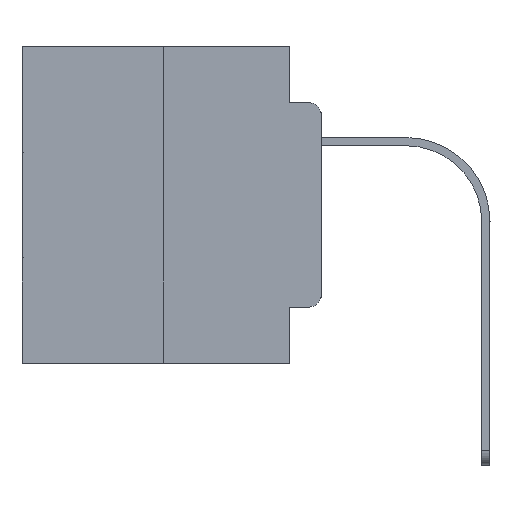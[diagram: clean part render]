
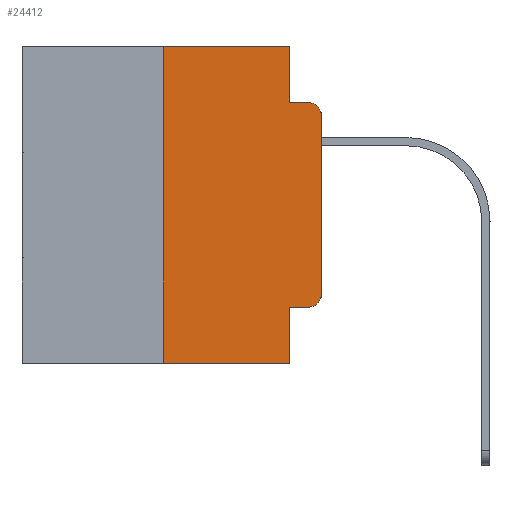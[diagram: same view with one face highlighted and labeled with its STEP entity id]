
A CAD part, left-side view. The second image highlights one B-rep face of the part: STEP entity #24412.
In plain terms, the highlighted planar face has unit normal (-1, 0, 0).
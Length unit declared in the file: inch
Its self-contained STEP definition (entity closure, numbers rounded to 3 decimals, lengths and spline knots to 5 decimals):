
#120 = CARTESIAN_POINT ( 'NONE',  ( 0., 0.051, -0.5 ) ) ;
#206 = ORIENTED_EDGE ( 'NONE', *, *, #8488, .T. ) ;
#531 = DIRECTION ( 'NONE',  ( 0., 0., -1. ) ) ;
#1294 = EDGE_CURVE ( 'NONE', #10812, #5511, #18435, .T. ) ;
#1433 = CARTESIAN_POINT ( 'NONE',  ( 0., 0.051, -0.4115 ) ) ;
#1598 = VERTEX_POINT ( 'NONE', #1433 ) ;
#1786 = CARTESIAN_POINT ( 'NONE',  ( 0., 0.02, -0.3915 ) ) ;
#2183 = DIRECTION ( 'NONE',  ( 1., 0., 0. ) ) ;
#2204 = DIRECTION ( 'NONE',  ( 0., 0., 1. ) ) ;
#2426 = VECTOR ( 'NONE', #15109, 39.37008 ) ;
#2468 = LINE ( 'NONE', #6788, #6600 ) ;
#2568 = DIRECTION ( 'NONE',  ( 0., -1., 0. ) ) ;
#2831 = DIRECTION ( 'NONE',  ( 0., -1., 0. ) ) ;
#2856 = LINE ( 'NONE', #23147, #14906 ) ;
#3822 = ORIENTED_EDGE ( 'NONE', *, *, #11584, .F. ) ;
#3892 = VERTEX_POINT ( 'NONE', #4068 ) ;
#4068 = CARTESIAN_POINT ( 'NONE',  ( 0., 0., -0.3915 ) ) ;
#4107 = DIRECTION ( 'NONE',  ( 0., 0., -1. ) ) ;
#4409 = VECTOR ( 'NONE', #6607, 39.37008 ) ;
#4613 = PLANE ( 'NONE',  #5698 ) ;
#5511 = VERTEX_POINT ( 'NONE', #15669 ) ;
#5698 = AXIS2_PLACEMENT_3D ( 'NONE', #10422, #2183, #10957 ) ;
#6008 = CARTESIAN_POINT ( 'NONE',  ( 0., 0.02, -0.1085 ) ) ;
#6032 = DIRECTION ( 'NONE',  ( 0., -1., 0. ) ) ;
#6600 = VECTOR ( 'NONE', #2204, 39.37008 ) ;
#6607 = DIRECTION ( 'NONE',  ( 0., 0., 1. ) ) ;
#6787 = EDGE_CURVE ( 'NONE', #10976, #25309, #18533, .T. ) ;
#6788 = CARTESIAN_POINT ( 'NONE',  ( 0., 0., 0. ) ) ;
#7060 = AXIS2_PLACEMENT_3D ( 'NONE', #6008, #7903, #4107 ) ;
#7903 = DIRECTION ( 'NONE',  ( -1., 0., 0. ) ) ;
#8488 = EDGE_CURVE ( 'NONE', #9969, #12125, #22486, .T. ) ;
#8764 = CARTESIAN_POINT ( 'NONE',  ( 0., 0.051, 0. ) ) ;
#8902 = EDGE_LOOP ( 'NONE', ( #17900, #206, #23940, #16121, #20036, #3822, #11712, #24834, #10517, #17631 ) ) ;
#9312 = LINE ( 'NONE', #17511, #2426 ) ;
#9969 = VERTEX_POINT ( 'NONE', #13968 ) ;
#10422 = CARTESIAN_POINT ( 'NONE',  ( 0., 0.473, 0. ) ) ;
#10517 = ORIENTED_EDGE ( 'NONE', *, *, #19918, .T. ) ;
#10812 = VERTEX_POINT ( 'NONE', #23879 ) ;
#10957 = DIRECTION ( 'NONE',  ( 0., 0., -1. ) ) ;
#10976 = VERTEX_POINT ( 'NONE', #13969 ) ;
#11100 = CARTESIAN_POINT ( 'NONE',  ( 0., 0.02, -0.4115 ) ) ;
#11236 = CIRCLE ( 'NONE', #21063, 0.02 ) ;
#11324 = VERTEX_POINT ( 'NONE', #19416 ) ;
#11584 = EDGE_CURVE ( 'NONE', #10976, #11324, #18857, .T. ) ;
#11661 = VECTOR ( 'NONE', #6032, 39.37008 ) ;
#11712 = ORIENTED_EDGE ( 'NONE', *, *, #6787, .T. ) ;
#12125 = VERTEX_POINT ( 'NONE', #23629 ) ;
#13400 = VECTOR ( 'NONE', #531, 39.37008 ) ;
#13942 = DIRECTION ( 'NONE',  ( -1., 0., 0. ) ) ;
#13968 = CARTESIAN_POINT ( 'NONE',  ( 0., 0., -0.1085 ) ) ;
#13969 = CARTESIAN_POINT ( 'NONE',  ( 0., 0.25, -0.5 ) ) ;
#14057 = VERTEX_POINT ( 'NONE', #11100 ) ;
#14059 = LINE ( 'NONE', #8764, #13400 ) ;
#14600 = EDGE_CURVE ( 'NONE', #3892, #9969, #2468, .T. ) ;
#14906 = VECTOR ( 'NONE', #2568, 39.37008 ) ;
#15109 = DIRECTION ( 'NONE',  ( 0., -1., 0. ) ) ;
#15669 = CARTESIAN_POINT ( 'NONE',  ( 0., 0.051, -0.0885 ) ) ;
#16121 = ORIENTED_EDGE ( 'NONE', *, *, #1294, .F. ) ;
#16690 = DIRECTION ( 'NONE',  ( 0., 0., -1. ) ) ;
#16880 = EDGE_CURVE ( 'NONE', #11324, #10812, #9312, .T. ) ;
#17511 = CARTESIAN_POINT ( 'NONE',  ( 0., 0.473, 0. ) ) ;
#17631 = ORIENTED_EDGE ( 'NONE', *, *, #22977, .T. ) ;
#17900 = ORIENTED_EDGE ( 'NONE', *, *, #14600, .T. ) ;
#18257 = EDGE_CURVE ( 'NONE', #5511, #12125, #2856, .T. ) ;
#18435 = LINE ( 'NONE', #20680, #21649 ) ;
#18533 = LINE ( 'NONE', #26464, #11661 ) ;
#18857 = LINE ( 'NONE', #20723, #4409 ) ;
#18967 = LINE ( 'NONE', #19107, #21801 ) ;
#19107 = CARTESIAN_POINT ( 'NONE',  ( 0., 0.051, -0.4115 ) ) ;
#19416 = CARTESIAN_POINT ( 'NONE',  ( 0., 0.25, 0. ) ) ;
#19918 = EDGE_CURVE ( 'NONE', #1598, #14057, #18967, .T. ) ;
#20036 = ORIENTED_EDGE ( 'NONE', *, *, #16880, .F. ) ;
#20680 = CARTESIAN_POINT ( 'NONE',  ( 0., 0.051, 0. ) ) ;
#20723 = CARTESIAN_POINT ( 'NONE',  ( 0., 0.25, 0. ) ) ;
#21063 = AXIS2_PLACEMENT_3D ( 'NONE', #1786, #13942, #26414 ) ;
#21649 = VECTOR ( 'NONE', #16690, 39.37008 ) ;
#21801 = VECTOR ( 'NONE', #2831, 39.37008 ) ;
#22486 = CIRCLE ( 'NONE', #7060, 0.02 ) ;
#22977 = EDGE_CURVE ( 'NONE', #14057, #3892, #11236, .T. ) ;
#23147 = CARTESIAN_POINT ( 'NONE',  ( 0., 0.051, -0.0885 ) ) ;
#23629 = CARTESIAN_POINT ( 'NONE',  ( 0., 0.02, -0.0885 ) ) ;
#23879 = CARTESIAN_POINT ( 'NONE',  ( 0., 0.051, 0. ) ) ;
#23940 = ORIENTED_EDGE ( 'NONE', *, *, #18257, .F. ) ;
#24412 = ADVANCED_FACE ( 'NONE', ( #24907 ), #4613, .F. ) ;
#24824 = EDGE_CURVE ( 'NONE', #1598, #25309, #14059, .T. ) ;
#24834 = ORIENTED_EDGE ( 'NONE', *, *, #24824, .F. ) ;
#24907 = FACE_OUTER_BOUND ( 'NONE', #8902, .T. ) ;
#25309 = VERTEX_POINT ( 'NONE', #120 ) ;
#26414 = DIRECTION ( 'NONE',  ( 0., 0., -1. ) ) ;
#26464 = CARTESIAN_POINT ( 'NONE',  ( 0., 0.473, -0.5 ) ) ;
